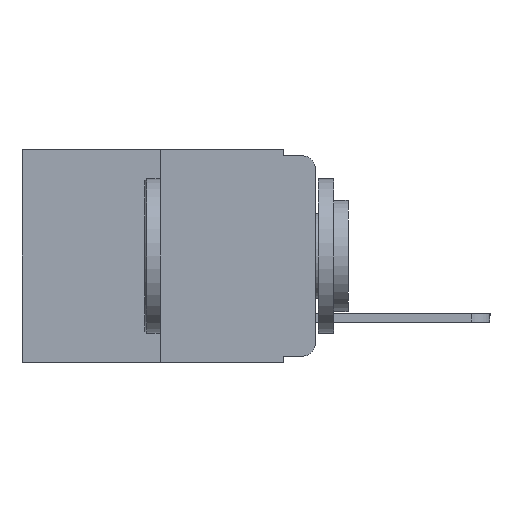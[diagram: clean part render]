
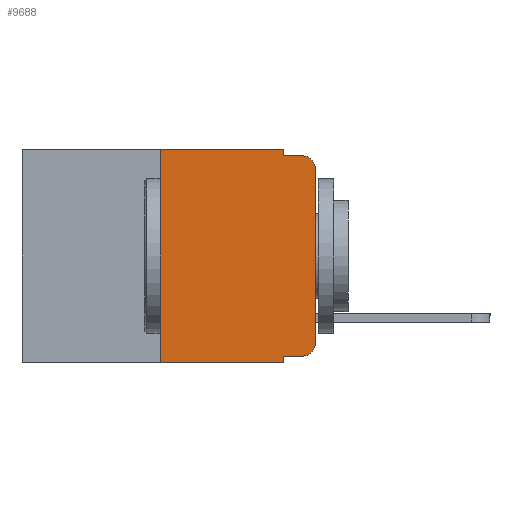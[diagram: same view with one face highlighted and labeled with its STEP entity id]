
A CAD part, left-side view. The second image highlights one B-rep face of the part: STEP entity #9688.
In plain terms, the highlighted planar face has unit normal (-1, 0, 0).
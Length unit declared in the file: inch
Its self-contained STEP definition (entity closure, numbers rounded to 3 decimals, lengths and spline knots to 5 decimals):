
#100 = EDGE_CURVE ( 'NONE', #10048, #10699, #9319, .T. ) ;
#195 = DIRECTION ( 'NONE',  ( 0., -1., 0. ) ) ;
#362 = VERTEX_POINT ( 'NONE', #11703 ) ;
#718 = CARTESIAN_POINT ( 'NONE',  ( 0., 0.473, -0.343 ) ) ;
#755 = CARTESIAN_POINT ( 'NONE',  ( 0., 0.25, 0. ) ) ;
#845 = CARTESIAN_POINT ( 'NONE',  ( 0., 0.473, 0. ) ) ;
#883 = DIRECTION ( 'NONE',  ( 0., -1., 0. ) ) ;
#891 = EDGE_CURVE ( 'NONE', #10048, #5609, #10210, .T. ) ;
#892 = DIRECTION ( 'NONE',  ( 0., 0., -1. ) ) ;
#1045 = ORIENTED_EDGE ( 'NONE', *, *, #891, .F. ) ;
#1235 = CARTESIAN_POINT ( 'NONE',  ( 0., 0., 0. ) ) ;
#1331 = VECTOR ( 'NONE', #4116, 39.37008 ) ;
#1392 = VERTEX_POINT ( 'NONE', #755 ) ;
#1485 = CIRCLE ( 'NONE', #8580, 0.02 ) ;
#1628 = VECTOR ( 'NONE', #195, 39.37008 ) ;
#1768 = CARTESIAN_POINT ( 'NONE',  ( 0., 0.25, -0.343 ) ) ;
#1841 = CARTESIAN_POINT ( 'NONE',  ( 0., 0.051, 0. ) ) ;
#1900 = EDGE_CURVE ( 'NONE', #6358, #1392, #4246, .T. ) ;
#2075 = DIRECTION ( 'NONE',  ( 0., 0., -1. ) ) ;
#2262 = ORIENTED_EDGE ( 'NONE', *, *, #2593, .T. ) ;
#2563 = CARTESIAN_POINT ( 'NONE',  ( 0., 0.051, -0.343 ) ) ;
#2593 = EDGE_CURVE ( 'NONE', #10699, #3193, #1485, .T. ) ;
#2796 = CARTESIAN_POINT ( 'NONE',  ( 0., 0., -0.313 ) ) ;
#2854 = LINE ( 'NONE', #10639, #7641 ) ;
#3193 = VERTEX_POINT ( 'NONE', #2796 ) ;
#3456 = CARTESIAN_POINT ( 'NONE',  ( 0., 0.02, -0.333 ) ) ;
#4063 = VERTEX_POINT ( 'NONE', #4326 ) ;
#4116 = DIRECTION ( 'NONE',  ( 0., 0., 1. ) ) ;
#4246 = LINE ( 'NONE', #4553, #8723 ) ;
#4326 = CARTESIAN_POINT ( 'NONE',  ( 0., 0.02, -0.01 ) ) ;
#4455 = ORIENTED_EDGE ( 'NONE', *, *, #11977, .F. ) ;
#4549 = EDGE_CURVE ( 'NONE', #1392, #362, #2854, .T. ) ;
#4553 = CARTESIAN_POINT ( 'NONE',  ( 0., 0.25, 0. ) ) ;
#4913 = CARTESIAN_POINT ( 'NONE',  ( 0., 0.051, -0.01 ) ) ;
#5132 = DIRECTION ( 'NONE',  ( 0., 0., 1. ) ) ;
#5200 = DIRECTION ( 'NONE',  ( -1., 0., 0. ) ) ;
#5362 = ORIENTED_EDGE ( 'NONE', *, *, #4549, .F. ) ;
#5474 = EDGE_LOOP ( 'NONE', ( #6844, #7743, #10883, #4455, #5362, #11631, #7758, #1045, #10165, #2262 ) ) ;
#5609 = VERTEX_POINT ( 'NONE', #2563 ) ;
#5614 = EDGE_CURVE ( 'NONE', #6358, #5609, #6595, .T. ) ;
#5819 = VERTEX_POINT ( 'NONE', #9506 ) ;
#5854 = CARTESIAN_POINT ( 'NONE',  ( 0., 0.051, 0. ) ) ;
#5963 = CARTESIAN_POINT ( 'NONE',  ( 0., 0.02, -0.313 ) ) ;
#5975 = FACE_OUTER_BOUND ( 'NONE', #5474, .T. ) ;
#6034 = EDGE_CURVE ( 'NONE', #3193, #8436, #8950, .T. ) ;
#6146 = CARTESIAN_POINT ( 'NONE',  ( 0., 0.051, -0.333 ) ) ;
#6358 = VERTEX_POINT ( 'NONE', #1768 ) ;
#6374 = VECTOR ( 'NONE', #8349, 39.37008 ) ;
#6595 = LINE ( 'NONE', #718, #6374 ) ;
#6598 = DIRECTION ( 'NONE',  ( 1., 0., 0. ) ) ;
#6844 = ORIENTED_EDGE ( 'NONE', *, *, #6034, .T. ) ;
#7276 = DIRECTION ( 'NONE',  ( 0., 0., -1. ) ) ;
#7450 = CIRCLE ( 'NONE', #10615, 0.02 ) ;
#7641 = VECTOR ( 'NONE', #10518, 39.37008 ) ;
#7661 = VECTOR ( 'NONE', #7276, 39.37008 ) ;
#7743 = ORIENTED_EDGE ( 'NONE', *, *, #10041, .T. ) ;
#7758 = ORIENTED_EDGE ( 'NONE', *, *, #5614, .T. ) ;
#8050 = CARTESIAN_POINT ( 'NONE',  ( 0., 0.051, -0.333 ) ) ;
#8349 = DIRECTION ( 'NONE',  ( 0., -1., 0. ) ) ;
#8436 = VERTEX_POINT ( 'NONE', #11514 ) ;
#8580 = AXIS2_PLACEMENT_3D ( 'NONE', #5963, #9925, #9942 ) ;
#8723 = VECTOR ( 'NONE', #5132, 39.37008 ) ;
#8915 = AXIS2_PLACEMENT_3D ( 'NONE', #845, #6598, #892 ) ;
#8950 = LINE ( 'NONE', #1235, #1331 ) ;
#9095 = VECTOR ( 'NONE', #2075, 39.37008 ) ;
#9319 = LINE ( 'NONE', #6146, #11564 ) ;
#9506 = CARTESIAN_POINT ( 'NONE',  ( 0., 0.051, -0.01 ) ) ;
#9688 = ADVANCED_FACE ( 'NONE', ( #5975 ), #10401, .F. ) ;
#9870 = EDGE_CURVE ( 'NONE', #5819, #4063, #11796, .T. ) ;
#9925 = DIRECTION ( 'NONE',  ( -1., 0., 0. ) ) ;
#9942 = DIRECTION ( 'NONE',  ( 0., 0., -1. ) ) ;
#10041 = EDGE_CURVE ( 'NONE', #8436, #4063, #7450, .T. ) ;
#10048 = VERTEX_POINT ( 'NONE', #8050 ) ;
#10165 = ORIENTED_EDGE ( 'NONE', *, *, #100, .T. ) ;
#10210 = LINE ( 'NONE', #1841, #7661 ) ;
#10401 = PLANE ( 'NONE',  #8915 ) ;
#10518 = DIRECTION ( 'NONE',  ( 0., -1., 0. ) ) ;
#10615 = AXIS2_PLACEMENT_3D ( 'NONE', #10933, #5200, #11877 ) ;
#10639 = CARTESIAN_POINT ( 'NONE',  ( 0., 0.473, 0. ) ) ;
#10699 = VERTEX_POINT ( 'NONE', #3456 ) ;
#10883 = ORIENTED_EDGE ( 'NONE', *, *, #9870, .F. ) ;
#10933 = CARTESIAN_POINT ( 'NONE',  ( 0., 0.02, -0.03 ) ) ;
#11514 = CARTESIAN_POINT ( 'NONE',  ( 0., 0., -0.03 ) ) ;
#11564 = VECTOR ( 'NONE', #883, 39.37008 ) ;
#11631 = ORIENTED_EDGE ( 'NONE', *, *, #1900, .F. ) ;
#11703 = CARTESIAN_POINT ( 'NONE',  ( 0., 0.051, 0. ) ) ;
#11796 = LINE ( 'NONE', #4913, #1628 ) ;
#11877 = DIRECTION ( 'NONE',  ( 0., 0., -1. ) ) ;
#11933 = LINE ( 'NONE', #5854, #9095 ) ;
#11977 = EDGE_CURVE ( 'NONE', #362, #5819, #11933, .T. ) ;
